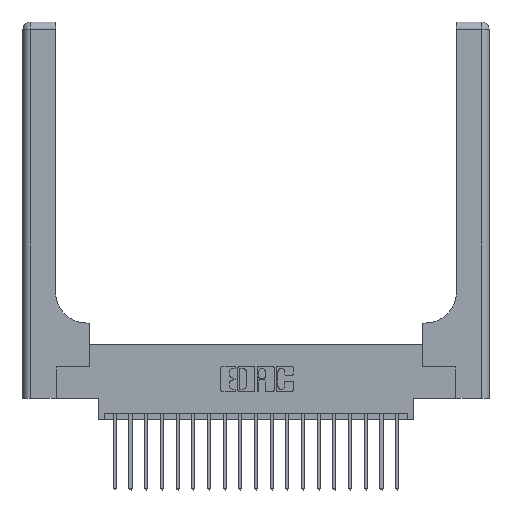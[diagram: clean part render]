
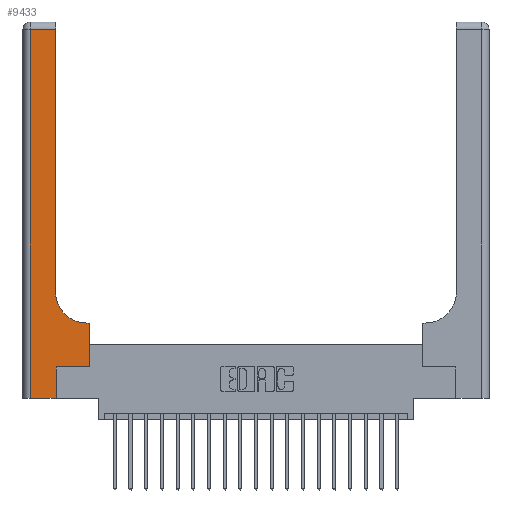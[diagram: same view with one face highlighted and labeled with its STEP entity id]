
A CAD part, top view. The second image highlights one B-rep face of the part: STEP entity #9433.
In plain terms, the highlighted planar face has unit normal (0, 0, 1).
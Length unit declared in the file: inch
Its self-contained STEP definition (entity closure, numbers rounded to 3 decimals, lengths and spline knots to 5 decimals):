
#21 = CARTESIAN_POINT ( 'NONE',  ( 0.528, 0.6, 0.37 ) ) ;
#257 = CARTESIAN_POINT ( 'NONE',  ( 0.265, 0.25, 0.37 ) ) ;
#376 = CARTESIAN_POINT ( 'NONE',  ( 0., 2.94, 0.37 ) ) ;
#392 = VERTEX_POINT ( 'NONE', #16062 ) ;
#433 = DIRECTION ( 'NONE',  ( 0., 1., 0. ) ) ;
#645 = DIRECTION ( 'NONE',  ( 1., 0., 0. ) ) ;
#1434 = ORIENTED_EDGE ( 'NONE', *, *, #9392, .T. ) ;
#1459 = VERTEX_POINT ( 'NONE', #257 ) ;
#1873 = LINE ( 'NONE', #376, #8812 ) ;
#2349 = CARTESIAN_POINT ( 'NONE',  ( 0., 0., 0.37 ) ) ;
#3377 = ORIENTED_EDGE ( 'NONE', *, *, #10208, .T. ) ;
#4940 = DIRECTION ( 'NONE',  ( 0., 0., -1. ) ) ;
#4954 = CARTESIAN_POINT ( 'NONE',  ( 0.26, 2.94, 0.37 ) ) ;
#5421 = LINE ( 'NONE', #11642, #13342 ) ;
#6058 = CARTESIAN_POINT ( 'NONE',  ( 0.06, 2.94, 0.37 ) ) ;
#6276 = CARTESIAN_POINT ( 'NONE',  ( 0.26, 0.6, 0.37 ) ) ;
#6414 = LINE ( 'NONE', #11556, #15473 ) ;
#6494 = CARTESIAN_POINT ( 'NONE',  ( 0.528, 0.25, 0.37 ) ) ;
#6549 = DIRECTION ( 'NONE',  ( 0., -1., 0. ) ) ;
#6703 = CARTESIAN_POINT ( 'NONE',  ( 0.528, 0.25, 0.37 ) ) ;
#7577 = EDGE_CURVE ( 'NONE', #15344, #392, #20997, .T. ) ;
#7901 = EDGE_CURVE ( 'NONE', #9533, #9191, #19142, .T. ) ;
#8191 = VERTEX_POINT ( 'NONE', #4954 ) ;
#8451 = DIRECTION ( 'NONE',  ( -1., 0., 0. ) ) ;
#8812 = VECTOR ( 'NONE', #8451, 39.37008 ) ;
#9191 = VERTEX_POINT ( 'NONE', #17513 ) ;
#9392 = EDGE_CURVE ( 'NONE', #10491, #9533, #9855, .T. ) ;
#9433 = ADVANCED_FACE ( 'NONE', ( #15028 ), #13112, .F. ) ;
#9533 = VERTEX_POINT ( 'NONE', #10390 ) ;
#9821 = EDGE_CURVE ( 'NONE', #1459, #18063, #6414, .T. ) ;
#9855 = LINE ( 'NONE', #16332, #19532 ) ;
#10208 = EDGE_CURVE ( 'NONE', #18063, #15344, #11530, .T. ) ;
#10390 = CARTESIAN_POINT ( 'NONE',  ( 0.06, 0., 0.37 ) ) ;
#10477 = ORIENTED_EDGE ( 'NONE', *, *, #11576, .T. ) ;
#10491 = VERTEX_POINT ( 'NONE', #6058 ) ;
#10937 = ORIENTED_EDGE ( 'NONE', *, *, #7901, .T. ) ;
#11530 = LINE ( 'NONE', #6703, #20804 ) ;
#11556 = CARTESIAN_POINT ( 'NONE',  ( 0.265, 0.25, 0.37 ) ) ;
#11576 = EDGE_CURVE ( 'NONE', #392, #15173, #12261, .T. ) ;
#11642 = CARTESIAN_POINT ( 'NONE',  ( 0.265, 0., 0.37 ) ) ;
#11668 = DIRECTION ( 'NONE',  ( 1., 0., 0. ) ) ;
#11753 = CARTESIAN_POINT ( 'NONE',  ( 0.51, 0.85, 0.37 ) ) ;
#12037 = EDGE_LOOP ( 'NONE', ( #15312, #14696, #1434, #10937, #13050, #16750, #3377, #15244, #10477 ) ) ;
#12261 = CIRCLE ( 'NONE', #17738, 0.25 ) ;
#12646 = CARTESIAN_POINT ( 'NONE',  ( 0.26, 0.85, 0.37 ) ) ;
#13050 = ORIENTED_EDGE ( 'NONE', *, *, #15400, .T. ) ;
#13112 = PLANE ( 'NONE',  #16113 ) ;
#13289 = DIRECTION ( 'NONE',  ( 0., 1., 0. ) ) ;
#13342 = VECTOR ( 'NONE', #433, 39.37008 ) ;
#13389 = EDGE_CURVE ( 'NONE', #8191, #10491, #1873, .T. ) ;
#13793 = VECTOR ( 'NONE', #13289, 39.37008 ) ;
#13886 = DIRECTION ( 'NONE',  ( 1., 0., 0. ) ) ;
#14696 = ORIENTED_EDGE ( 'NONE', *, *, #13389, .T. ) ;
#14699 = VECTOR ( 'NONE', #19275, 39.37008 ) ;
#15028 = FACE_OUTER_BOUND ( 'NONE', #12037, .T. ) ;
#15173 = VERTEX_POINT ( 'NONE', #12646 ) ;
#15244 = ORIENTED_EDGE ( 'NONE', *, *, #7577, .T. ) ;
#15312 = ORIENTED_EDGE ( 'NONE', *, *, #18919, .T. ) ;
#15344 = VERTEX_POINT ( 'NONE', #21 ) ;
#15400 = EDGE_CURVE ( 'NONE', #9191, #1459, #5421, .T. ) ;
#15473 = VECTOR ( 'NONE', #11668, 39.37008 ) ;
#16062 = CARTESIAN_POINT ( 'NONE',  ( 0.51, 0.6, 0.37 ) ) ;
#16113 = AXIS2_PLACEMENT_3D ( 'NONE', #19662, #4940, #19557 ) ;
#16332 = CARTESIAN_POINT ( 'NONE',  ( 0.06, 3., 0.37 ) ) ;
#16750 = ORIENTED_EDGE ( 'NONE', *, *, #9821, .T. ) ;
#17513 = CARTESIAN_POINT ( 'NONE',  ( 0.265, 0., 0.37 ) ) ;
#17738 = AXIS2_PLACEMENT_3D ( 'NONE', #11753, #20244, #645 ) ;
#17862 = VECTOR ( 'NONE', #13886, 39.37008 ) ;
#18063 = VERTEX_POINT ( 'NONE', #6494 ) ;
#18329 = LINE ( 'NONE', #20266, #13793 ) ;
#18919 = EDGE_CURVE ( 'NONE', #15173, #8191, #18329, .T. ) ;
#19142 = LINE ( 'NONE', #2349, #17862 ) ;
#19275 = DIRECTION ( 'NONE',  ( -1., 0., 0. ) ) ;
#19391 = DIRECTION ( 'NONE',  ( 0., 1., 0. ) ) ;
#19532 = VECTOR ( 'NONE', #6549, 39.37008 ) ;
#19557 = DIRECTION ( 'NONE',  ( -1., 0., 0. ) ) ;
#19662 = CARTESIAN_POINT ( 'NONE',  ( 0., 3., 0.37 ) ) ;
#20244 = DIRECTION ( 'NONE',  ( 0., 0., -1. ) ) ;
#20266 = CARTESIAN_POINT ( 'NONE',  ( 0.26, 3., 0.37 ) ) ;
#20804 = VECTOR ( 'NONE', #19391, 39.37008 ) ;
#20997 = LINE ( 'NONE', #6276, #14699 ) ;
